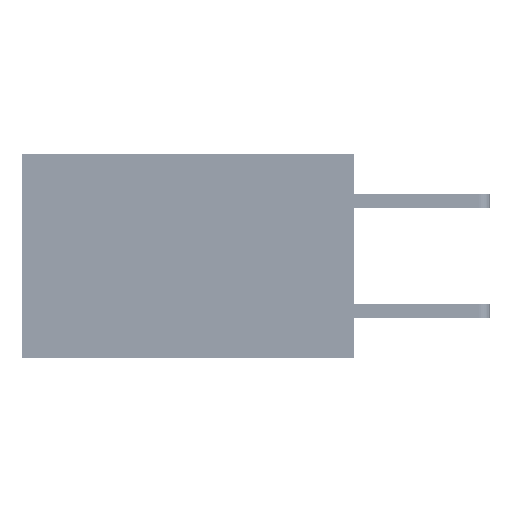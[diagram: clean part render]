
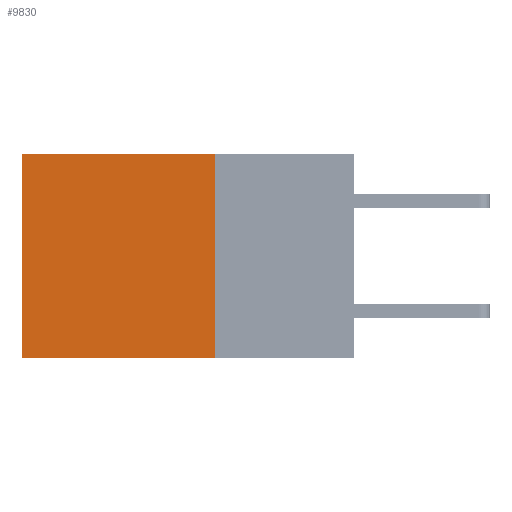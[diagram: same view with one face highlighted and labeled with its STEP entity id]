
A CAD part, left-side view. The second image highlights one B-rep face of the part: STEP entity #9830.
In plain terms, the highlighted planar face has unit normal (-1, 0, 0).
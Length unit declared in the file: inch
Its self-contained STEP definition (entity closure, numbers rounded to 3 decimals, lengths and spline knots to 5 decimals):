
#853 = LINE ( 'NONE', #48112, #16133 ) ;
#1841 = VERTEX_POINT ( 'NONE', #22492 ) ;
#2183 = PLANE ( 'NONE',  #39149 ) ;
#2839 = VERTEX_POINT ( 'NONE', #30625 ) ;
#4907 = VERTEX_POINT ( 'NONE', #22008 ) ;
#6506 = VECTOR ( 'NONE', #29961, 39.37008 ) ;
#9830 = ADVANCED_FACE ( 'NONE', ( #13287 ), #2183, .F. ) ;
#13023 = VECTOR ( 'NONE', #29088, 39.37008 ) ;
#13287 = FACE_OUTER_BOUND ( 'NONE', #50490, .T. ) ;
#14184 = CARTESIAN_POINT ( 'NONE',  ( 0.2875, 0.25, -0.37 ) ) ;
#16133 = VECTOR ( 'NONE', #40361, 39.37008 ) ;
#16303 = ORIENTED_EDGE ( 'NONE', *, *, #18224, .F. ) ;
#18224 = EDGE_CURVE ( 'NONE', #2839, #29792, #853, .T. ) ;
#18324 = LINE ( 'NONE', #14184, #6506 ) ;
#18488 = CARTESIAN_POINT ( 'NONE',  ( 0.2875, 0.6, 0. ) ) ;
#20298 = CARTESIAN_POINT ( 'NONE',  ( 0.2875, 0.25, -0.37 ) ) ;
#20553 = LINE ( 'NONE', #36316, #13023 ) ;
#20896 = EDGE_CURVE ( 'NONE', #2839, #4907, #20553, .T. ) ;
#22008 = CARTESIAN_POINT ( 'NONE',  ( 0.2875, 0.6, 0. ) ) ;
#22200 = EDGE_CURVE ( 'NONE', #29792, #1841, #18324, .T. ) ;
#22492 = CARTESIAN_POINT ( 'NONE',  ( 0.2875, 0.6, -0.37 ) ) ;
#26209 = DIRECTION ( 'NONE',  ( 0., 0., -1. ) ) ;
#26934 = ORIENTED_EDGE ( 'NONE', *, *, #40543, .T. ) ;
#27276 = VECTOR ( 'NONE', #45864, 39.37008 ) ;
#29088 = DIRECTION ( 'NONE',  ( 0., 1., 0. ) ) ;
#29792 = VERTEX_POINT ( 'NONE', #20298 ) ;
#29961 = DIRECTION ( 'NONE',  ( 0., 1., 0. ) ) ;
#30127 = LINE ( 'NONE', #18488, #27276 ) ;
#30625 = CARTESIAN_POINT ( 'NONE',  ( 0.2875, 0.25, 0. ) ) ;
#32730 = ORIENTED_EDGE ( 'NONE', *, *, #22200, .F. ) ;
#32928 = DIRECTION ( 'NONE',  ( 1., 0., 0. ) ) ;
#33687 = CARTESIAN_POINT ( 'NONE',  ( 0.2875, 0.25, 0. ) ) ;
#36316 = CARTESIAN_POINT ( 'NONE',  ( 0.2875, 0.25, 0. ) ) ;
#39149 = AXIS2_PLACEMENT_3D ( 'NONE', #33687, #32928, #26209 ) ;
#40361 = DIRECTION ( 'NONE',  ( 0., 0., -1. ) ) ;
#40543 = EDGE_CURVE ( 'NONE', #4907, #1841, #30127, .T. ) ;
#45864 = DIRECTION ( 'NONE',  ( 0., 0., -1. ) ) ;
#47219 = ORIENTED_EDGE ( 'NONE', *, *, #20896, .T. ) ;
#48112 = CARTESIAN_POINT ( 'NONE',  ( 0.2875, 0.25, 0. ) ) ;
#50490 = EDGE_LOOP ( 'NONE', ( #26934, #32730, #16303, #47219 ) ) ;
